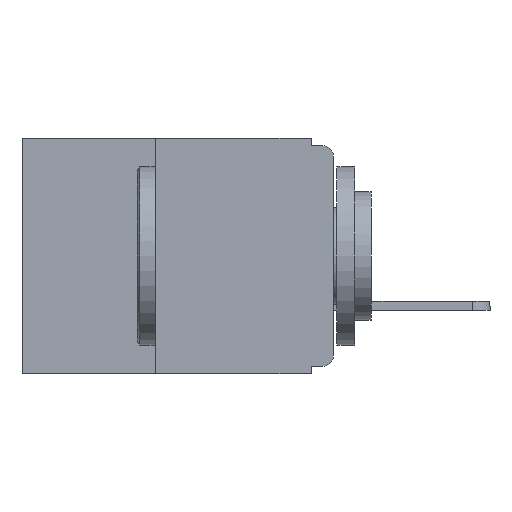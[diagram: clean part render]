
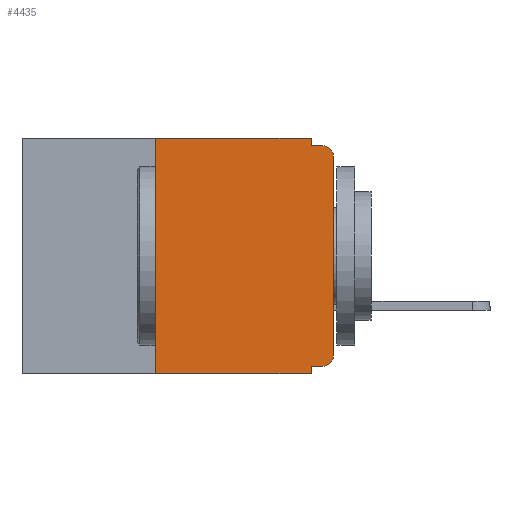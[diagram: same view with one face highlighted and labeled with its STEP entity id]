
A CAD part, left-side view. The second image highlights one B-rep face of the part: STEP entity #4435.
In plain terms, the highlighted planar face has unit normal (-1, 0, 0).
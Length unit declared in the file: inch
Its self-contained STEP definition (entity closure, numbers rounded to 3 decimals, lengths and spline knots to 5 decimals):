
#1091 = VERTEX_POINT ( 'NONE', #9220 ) ;
#1315 = CARTESIAN_POINT ( 'NONE',  ( 0., 0.031, -0.01 ) ) ;
#1397 = LINE ( 'NONE', #9858, #1467 ) ;
#1433 = VERTEX_POINT ( 'NONE', #11207 ) ;
#1467 = VECTOR ( 'NONE', #8698, 39.37008 ) ;
#1719 = VECTOR ( 'NONE', #8364, 39.37008 ) ;
#2414 = VERTEX_POINT ( 'NONE', #1315 ) ;
#3887 = VERTEX_POINT ( 'NONE', #9101 ) ;
#4435 = ADVANCED_FACE ( 'NONE', ( #11854 ), #15680, .F. ) ;
#4582 = VECTOR ( 'NONE', #8270, 39.37008 ) ;
#4605 = LINE ( 'NONE', #8660, #4582 ) ;
#4701 = VERTEX_POINT ( 'NONE', #10681 ) ;
#5147 = CARTESIAN_POINT ( 'NONE',  ( 0., 0., -0.305 ) ) ;
#5383 = VECTOR ( 'NONE', #7173, 39.37008 ) ;
#5411 = VERTEX_POINT ( 'NONE', #10919 ) ;
#5515 = LINE ( 'NONE', #7202, #5383 ) ;
#5568 = CARTESIAN_POINT ( 'NONE',  ( 0., 0.015, -0.01 ) ) ;
#6722 = EDGE_CURVE ( 'NONE', #18025, #1091, #5515, .T. ) ;
#7173 = DIRECTION ( 'NONE',  ( 0., 0., 1. ) ) ;
#7202 = CARTESIAN_POINT ( 'NONE',  ( 0., 0., 0. ) ) ;
#7358 = DIRECTION ( 'NONE',  ( 0., 0., -1. ) ) ;
#7404 = CARTESIAN_POINT ( 'NONE',  ( 0., 0.031, -0.33 ) ) ;
#7839 = EDGE_CURVE ( 'NONE', #3887, #1433, #1397, .T. ) ;
#8270 = DIRECTION ( 'NONE',  ( 0., -1., 0. ) ) ;
#8364 = DIRECTION ( 'NONE',  ( 0., 0., -1. ) ) ;
#8660 = CARTESIAN_POINT ( 'NONE',  ( 0., 0., -0.01 ) ) ;
#8698 = DIRECTION ( 'NONE',  ( 0., 1., 0. ) ) ;
#8735 = CARTESIAN_POINT ( 'NONE',  ( 0., 0.031, 0. ) ) ;
#9101 = CARTESIAN_POINT ( 'NONE',  ( 0., 0.015, -0.32 ) ) ;
#9220 = CARTESIAN_POINT ( 'NONE',  ( 0., 0., -0.025 ) ) ;
#9280 = VECTOR ( 'NONE', #17230, 39.37008 ) ;
#9357 = LINE ( 'NONE', #16861, #9280 ) ;
#9423 = CIRCLE ( 'NONE', #19124, 0.015 ) ;
#9449 = ORIENTED_EDGE ( 'NONE', *, *, #6722, .T. ) ;
#9510 = EDGE_LOOP ( 'NONE', ( #9449, #9565, #10201, #10273, #10534, #10609, #11209, #11267, #11404, #11496 ) ) ;
#9565 = ORIENTED_EDGE ( 'NONE', *, *, #9837, .T. ) ;
#9837 = EDGE_CURVE ( 'NONE', #1091, #15203, #15795, .T. ) ;
#9858 = CARTESIAN_POINT ( 'NONE',  ( 0., 0., -0.32 ) ) ;
#10201 = ORIENTED_EDGE ( 'NONE', *, *, #12549, .F. ) ;
#10273 = ORIENTED_EDGE ( 'NONE', *, *, #18356, .F. ) ;
#10534 = ORIENTED_EDGE ( 'NONE', *, *, #14987, .F. ) ;
#10609 = ORIENTED_EDGE ( 'NONE', *, *, #18236, .F. ) ;
#10681 = CARTESIAN_POINT ( 'NONE',  ( 0., 0.25, -0.33 ) ) ;
#10919 = CARTESIAN_POINT ( 'NONE',  ( 0., 0.031, 0. ) ) ;
#11207 = CARTESIAN_POINT ( 'NONE',  ( 0., 0.031, -0.32 ) ) ;
#11209 = ORIENTED_EDGE ( 'NONE', *, *, #18207, .T. ) ;
#11267 = ORIENTED_EDGE ( 'NONE', *, *, #18029, .F. ) ;
#11328 = EDGE_CURVE ( 'NONE', #3887, #18025, #9423, .T. ) ;
#11404 = ORIENTED_EDGE ( 'NONE', *, *, #7839, .F. ) ;
#11496 = ORIENTED_EDGE ( 'NONE', *, *, #11328, .T. ) ;
#11498 = VERTEX_POINT ( 'NONE', #12351 ) ;
#11791 = LINE ( 'NONE', #8735, #1719 ) ;
#11854 = FACE_OUTER_BOUND ( 'NONE', #9510, .T. ) ;
#11906 = DIRECTION ( 'NONE',  ( 0., 0., -1. ) ) ;
#12041 = DIRECTION ( 'NONE',  ( -1., 0., 0. ) ) ;
#12057 = CARTESIAN_POINT ( 'NONE',  ( 0., 0.015, -0.025 ) ) ;
#12133 = VECTOR ( 'NONE', #12335, 39.37008 ) ;
#12200 = CARTESIAN_POINT ( 'NONE',  ( 0., 0.25, -0.33 ) ) ;
#12216 = LINE ( 'NONE', #12200, #12133 ) ;
#12335 = DIRECTION ( 'NONE',  ( 0., 0., 1. ) ) ;
#12351 = CARTESIAN_POINT ( 'NONE',  ( 0., 0.031, -0.33 ) ) ;
#12414 = VECTOR ( 'NONE', #15032, 39.37008 ) ;
#12549 = EDGE_CURVE ( 'NONE', #2414, #15203, #4605, .T. ) ;
#12581 = LINE ( 'NONE', #15645, #12414 ) ;
#12854 = AXIS2_PLACEMENT_3D ( 'NONE', #12057, #12041, #11906 ) ;
#13130 = VERTEX_POINT ( 'NONE', #18140 ) ;
#13538 = VECTOR ( 'NONE', #7358, 39.37008 ) ;
#13859 = LINE ( 'NONE', #7404, #13538 ) ;
#14213 = AXIS2_PLACEMENT_3D ( 'NONE', #15704, #15840, #15612 ) ;
#14987 = EDGE_CURVE ( 'NONE', #13130, #5411, #9357, .T. ) ;
#15032 = DIRECTION ( 'NONE',  ( 0., -1., 0. ) ) ;
#15203 = VERTEX_POINT ( 'NONE', #5568 ) ;
#15612 = DIRECTION ( 'NONE',  ( 0., 0., -1. ) ) ;
#15645 = CARTESIAN_POINT ( 'NONE',  ( 0., 0.437, -0.33 ) ) ;
#15680 = PLANE ( 'NONE',  #14213 ) ;
#15704 = CARTESIAN_POINT ( 'NONE',  ( 0., 0.437, 0. ) ) ;
#15795 = CIRCLE ( 'NONE', #12854, 0.015 ) ;
#15840 = DIRECTION ( 'NONE',  ( 1., 0., 0. ) ) ;
#16861 = CARTESIAN_POINT ( 'NONE',  ( 0., 0.437, 0. ) ) ;
#17060 = DIRECTION ( 'NONE',  ( 0., 0., -1. ) ) ;
#17078 = DIRECTION ( 'NONE',  ( -1., 0., 0. ) ) ;
#17084 = CARTESIAN_POINT ( 'NONE',  ( 0., 0.015, -0.305 ) ) ;
#17230 = DIRECTION ( 'NONE',  ( 0., -1., 0. ) ) ;
#18025 = VERTEX_POINT ( 'NONE', #5147 ) ;
#18029 = EDGE_CURVE ( 'NONE', #1433, #11498, #13859, .T. ) ;
#18140 = CARTESIAN_POINT ( 'NONE',  ( 0., 0.25, 0. ) ) ;
#18207 = EDGE_CURVE ( 'NONE', #4701, #11498, #12581, .T. ) ;
#18236 = EDGE_CURVE ( 'NONE', #4701, #13130, #12216, .T. ) ;
#18356 = EDGE_CURVE ( 'NONE', #5411, #2414, #11791, .T. ) ;
#19124 = AXIS2_PLACEMENT_3D ( 'NONE', #17084, #17078, #17060 ) ;
